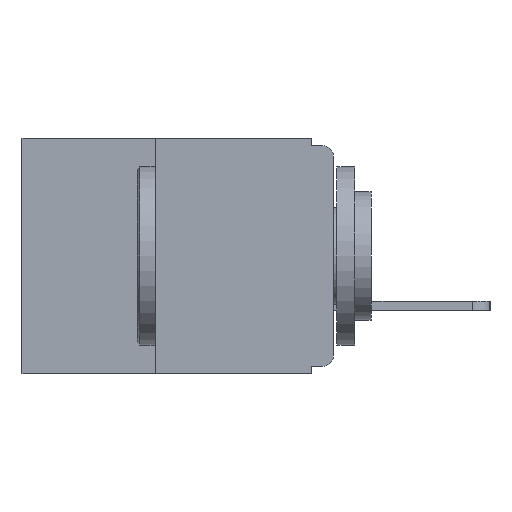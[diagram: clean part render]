
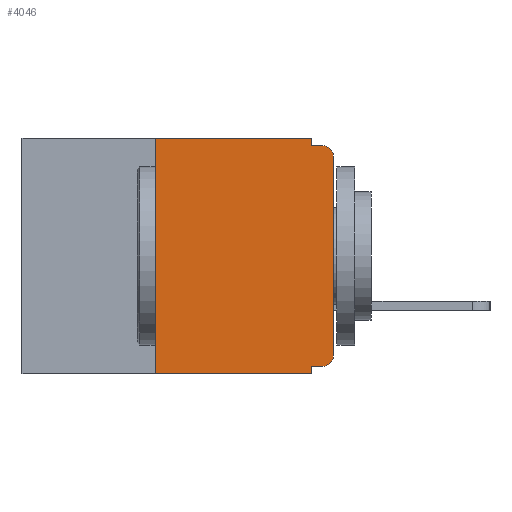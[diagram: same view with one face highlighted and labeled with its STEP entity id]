
A CAD part, left-side view. The second image highlights one B-rep face of the part: STEP entity #4046.
In plain terms, the highlighted planar face has unit normal (-1, 0, 0).
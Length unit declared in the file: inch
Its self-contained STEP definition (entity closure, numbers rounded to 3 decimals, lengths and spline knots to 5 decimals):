
#392 = CARTESIAN_POINT ( 'NONE',  ( 0., 0.015, -0.025 ) ) ;
#475 = CARTESIAN_POINT ( 'NONE',  ( 0., 0.031, 0. ) ) ;
#506 = DIRECTION ( 'NONE',  ( 0., -1., 0. ) ) ;
#719 = ORIENTED_EDGE ( 'NONE', *, *, #940, .F. ) ;
#935 = EDGE_CURVE ( 'NONE', #3042, #9532, #10373, .T. ) ;
#940 = EDGE_CURVE ( 'NONE', #13750, #6259, #5632, .T. ) ;
#1177 = DIRECTION ( 'NONE',  ( 1., 0., 0. ) ) ;
#1520 = VECTOR ( 'NONE', #11053, 39.37008 ) ;
#1719 = DIRECTION ( 'NONE',  ( 0., 0., -1. ) ) ;
#1750 = VERTEX_POINT ( 'NONE', #15725 ) ;
#2052 = ORIENTED_EDGE ( 'NONE', *, *, #9243, .F. ) ;
#2131 = CARTESIAN_POINT ( 'NONE',  ( 0., 0.015, -0.32 ) ) ;
#2199 = ORIENTED_EDGE ( 'NONE', *, *, #4927, .F. ) ;
#2256 = VERTEX_POINT ( 'NONE', #3978 ) ;
#2288 = VECTOR ( 'NONE', #16149, 39.37008 ) ;
#2433 = VECTOR ( 'NONE', #5774, 39.37008 ) ;
#3042 = VERTEX_POINT ( 'NONE', #12737 ) ;
#3364 = EDGE_CURVE ( 'NONE', #13750, #11423, #10705, .T. ) ;
#3645 = ORIENTED_EDGE ( 'NONE', *, *, #7097, .F. ) ;
#3679 = VERTEX_POINT ( 'NONE', #13064 ) ;
#3900 = FACE_OUTER_BOUND ( 'NONE', #7834, .T. ) ;
#3943 = CARTESIAN_POINT ( 'NONE',  ( 0., 0.25, -0.33 ) ) ;
#3978 = CARTESIAN_POINT ( 'NONE',  ( 0., 0.031, -0.01 ) ) ;
#3979 = CARTESIAN_POINT ( 'NONE',  ( 0., 0.015, -0.305 ) ) ;
#4046 = ADVANCED_FACE ( 'NONE', ( #3900 ), #11620, .F. ) ;
#4497 = CARTESIAN_POINT ( 'NONE',  ( 0., 0.25, -0.33 ) ) ;
#4590 = EDGE_CURVE ( 'NONE', #7321, #3042, #10457, .T. ) ;
#4609 = VECTOR ( 'NONE', #7540, 39.37008 ) ;
#4693 = VECTOR ( 'NONE', #10600, 39.37008 ) ;
#4862 = ORIENTED_EDGE ( 'NONE', *, *, #11041, .F. ) ;
#4927 = EDGE_CURVE ( 'NONE', #2256, #3679, #12360, .T. ) ;
#5632 = LINE ( 'NONE', #4497, #8520 ) ;
#5688 = DIRECTION ( 'NONE',  ( 0., 0., -1. ) ) ;
#5774 = DIRECTION ( 'NONE',  ( 0., -1., 0. ) ) ;
#5802 = CARTESIAN_POINT ( 'NONE',  ( 0., 0.031, 0. ) ) ;
#5806 = DIRECTION ( 'NONE',  ( -1., 0., 0. ) ) ;
#5826 = EDGE_CURVE ( 'NONE', #1750, #11423, #13175, .T. ) ;
#5920 = LINE ( 'NONE', #8339, #2433 ) ;
#6236 = CARTESIAN_POINT ( 'NONE',  ( 0., 0., -0.32 ) ) ;
#6259 = VERTEX_POINT ( 'NONE', #15548 ) ;
#6772 = VECTOR ( 'NONE', #1719, 39.37008 ) ;
#7097 = EDGE_CURVE ( 'NONE', #6259, #15944, #5920, .T. ) ;
#7153 = CARTESIAN_POINT ( 'NONE',  ( 0., 0.031, -0.33 ) ) ;
#7321 = VERTEX_POINT ( 'NONE', #2131 ) ;
#7540 = DIRECTION ( 'NONE',  ( 0., 1., 0. ) ) ;
#7831 = CARTESIAN_POINT ( 'NONE',  ( 0., 0., -0.01 ) ) ;
#7834 = EDGE_LOOP ( 'NONE', ( #10861, #11771, #2199, #4862, #3645, #719, #9744, #13539, #2052, #12189 ) ) ;
#7849 = CARTESIAN_POINT ( 'NONE',  ( 0., 0.437, 0. ) ) ;
#8339 = CARTESIAN_POINT ( 'NONE',  ( 0., 0.437, 0. ) ) ;
#8520 = VECTOR ( 'NONE', #11111, 39.37008 ) ;
#9060 = DIRECTION ( 'NONE',  ( 0., 0., -1. ) ) ;
#9149 = DIRECTION ( 'NONE',  ( 0., 0., -1. ) ) ;
#9243 = EDGE_CURVE ( 'NONE', #7321, #1750, #14297, .T. ) ;
#9532 = VERTEX_POINT ( 'NONE', #14853 ) ;
#9744 = ORIENTED_EDGE ( 'NONE', *, *, #3364, .T. ) ;
#10288 = VECTOR ( 'NONE', #506, 39.37008 ) ;
#10373 = LINE ( 'NONE', #13604, #1520 ) ;
#10457 = CIRCLE ( 'NONE', #12488, 0.015 ) ;
#10600 = DIRECTION ( 'NONE',  ( 0., -1., 0. ) ) ;
#10702 = AXIS2_PLACEMENT_3D ( 'NONE', #392, #5806, #5688 ) ;
#10705 = LINE ( 'NONE', #15041, #10288 ) ;
#10861 = ORIENTED_EDGE ( 'NONE', *, *, #935, .T. ) ;
#10909 = AXIS2_PLACEMENT_3D ( 'NONE', #7849, #1177, #9060 ) ;
#11041 = EDGE_CURVE ( 'NONE', #15944, #2256, #11561, .T. ) ;
#11053 = DIRECTION ( 'NONE',  ( 0., 0., 1. ) ) ;
#11111 = DIRECTION ( 'NONE',  ( 0., 0., 1. ) ) ;
#11423 = VERTEX_POINT ( 'NONE', #7153 ) ;
#11561 = LINE ( 'NONE', #5802, #2288 ) ;
#11572 = CIRCLE ( 'NONE', #10702, 0.015 ) ;
#11620 = PLANE ( 'NONE',  #10909 ) ;
#11771 = ORIENTED_EDGE ( 'NONE', *, *, #15078, .T. ) ;
#12189 = ORIENTED_EDGE ( 'NONE', *, *, #4590, .T. ) ;
#12360 = LINE ( 'NONE', #7831, #4693 ) ;
#12488 = AXIS2_PLACEMENT_3D ( 'NONE', #3979, #14519, #9149 ) ;
#12737 = CARTESIAN_POINT ( 'NONE',  ( 0., 0., -0.305 ) ) ;
#13064 = CARTESIAN_POINT ( 'NONE',  ( 0., 0.015, -0.01 ) ) ;
#13175 = LINE ( 'NONE', #16157, #6772 ) ;
#13539 = ORIENTED_EDGE ( 'NONE', *, *, #5826, .F. ) ;
#13604 = CARTESIAN_POINT ( 'NONE',  ( 0., 0., 0. ) ) ;
#13750 = VERTEX_POINT ( 'NONE', #3943 ) ;
#14297 = LINE ( 'NONE', #6236, #4609 ) ;
#14519 = DIRECTION ( 'NONE',  ( -1., 0., 0. ) ) ;
#14853 = CARTESIAN_POINT ( 'NONE',  ( 0., 0., -0.025 ) ) ;
#15041 = CARTESIAN_POINT ( 'NONE',  ( 0., 0.437, -0.33 ) ) ;
#15078 = EDGE_CURVE ( 'NONE', #9532, #3679, #11572, .T. ) ;
#15548 = CARTESIAN_POINT ( 'NONE',  ( 0., 0.25, 0. ) ) ;
#15725 = CARTESIAN_POINT ( 'NONE',  ( 0., 0.031, -0.32 ) ) ;
#15944 = VERTEX_POINT ( 'NONE', #475 ) ;
#16149 = DIRECTION ( 'NONE',  ( 0., 0., -1. ) ) ;
#16157 = CARTESIAN_POINT ( 'NONE',  ( 0., 0.031, -0.33 ) ) ;
